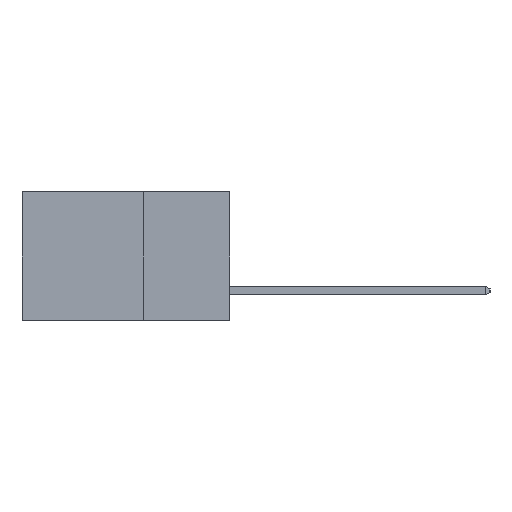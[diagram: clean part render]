
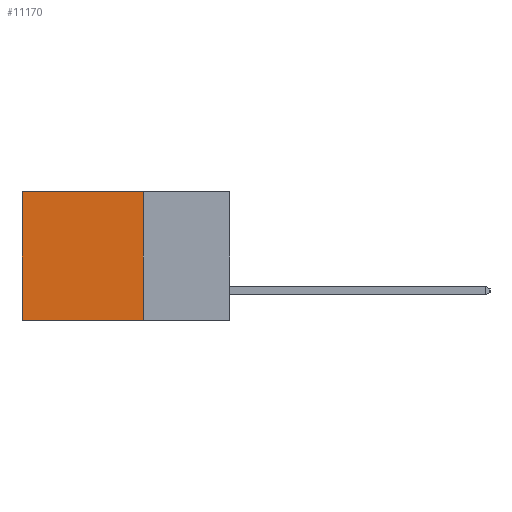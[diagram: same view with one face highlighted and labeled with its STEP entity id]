
A CAD part, left-side view. The second image highlights one B-rep face of the part: STEP entity #11170.
In plain terms, the highlighted planar face has unit normal (-1, 0, 0).
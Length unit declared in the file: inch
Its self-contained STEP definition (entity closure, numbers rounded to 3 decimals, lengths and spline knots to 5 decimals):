
#1221 = VERTEX_POINT ( 'NONE', #3160 ) ;
#1787 = CARTESIAN_POINT ( 'NONE',  ( 0.2615, 0.25, -0.37 ) ) ;
#2262 = VECTOR ( 'NONE', #6060, 39.37008 ) ;
#2928 = CARTESIAN_POINT ( 'NONE',  ( 0.2615, 0.6, -0.37 ) ) ;
#3160 = CARTESIAN_POINT ( 'NONE',  ( 0.2615, 0.25, 0. ) ) ;
#3195 = EDGE_CURVE ( 'NONE', #1221, #4773, #6312, .T. ) ;
#3609 = VECTOR ( 'NONE', #5332, 39.37008 ) ;
#3724 = EDGE_LOOP ( 'NONE', ( #5452, #7710, #10992, #6918 ) ) ;
#3962 = VECTOR ( 'NONE', #5372, 39.37008 ) ;
#4773 = VERTEX_POINT ( 'NONE', #9313 ) ;
#4808 = CARTESIAN_POINT ( 'NONE',  ( 0.2615, 0.25, -0.37 ) ) ;
#4959 = AXIS2_PLACEMENT_3D ( 'NONE', #4808, #11330, #5742 ) ;
#5332 = DIRECTION ( 'NONE',  ( 0., 1., 0. ) ) ;
#5372 = DIRECTION ( 'NONE',  ( 0., 0., -1. ) ) ;
#5404 = CARTESIAN_POINT ( 'NONE',  ( 0.2615, 0.25, -0.37 ) ) ;
#5452 = ORIENTED_EDGE ( 'NONE', *, *, #8070, .T. ) ;
#5742 = DIRECTION ( 'NONE',  ( 0., 0., -1. ) ) ;
#5817 = FACE_OUTER_BOUND ( 'NONE', #3724, .T. ) ;
#6060 = DIRECTION ( 'NONE',  ( 0., 0., -1. ) ) ;
#6312 = LINE ( 'NONE', #8985, #8211 ) ;
#6382 = EDGE_CURVE ( 'NONE', #1221, #10450, #6958, .T. ) ;
#6390 = LINE ( 'NONE', #5404, #3609 ) ;
#6440 = EDGE_CURVE ( 'NONE', #10450, #7061, #6390, .T. ) ;
#6583 = CARTESIAN_POINT ( 'NONE',  ( 0.2615, 0.25, -0.37 ) ) ;
#6918 = ORIENTED_EDGE ( 'NONE', *, *, #3195, .T. ) ;
#6958 = LINE ( 'NONE', #6583, #2262 ) ;
#7061 = VERTEX_POINT ( 'NONE', #2928 ) ;
#7583 = PLANE ( 'NONE',  #4959 ) ;
#7710 = ORIENTED_EDGE ( 'NONE', *, *, #6440, .F. ) ;
#8070 = EDGE_CURVE ( 'NONE', #4773, #7061, #8635, .T. ) ;
#8211 = VECTOR ( 'NONE', #8478, 39.37008 ) ;
#8478 = DIRECTION ( 'NONE',  ( 0., 1., 0. ) ) ;
#8635 = LINE ( 'NONE', #10955, #3962 ) ;
#8985 = CARTESIAN_POINT ( 'NONE',  ( 0.2615, 0.25, 0. ) ) ;
#9313 = CARTESIAN_POINT ( 'NONE',  ( 0.2615, 0.6, 0. ) ) ;
#10450 = VERTEX_POINT ( 'NONE', #1787 ) ;
#10955 = CARTESIAN_POINT ( 'NONE',  ( 0.2615, 0.6, -0.37 ) ) ;
#10992 = ORIENTED_EDGE ( 'NONE', *, *, #6382, .F. ) ;
#11170 = ADVANCED_FACE ( 'NONE', ( #5817 ), #7583, .F. ) ;
#11330 = DIRECTION ( 'NONE',  ( 1., 0., 0. ) ) ;
